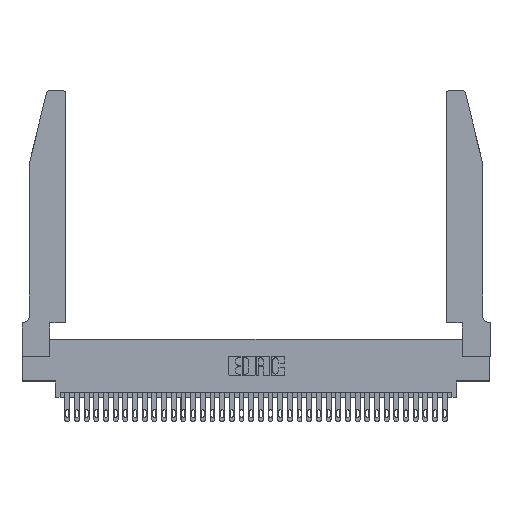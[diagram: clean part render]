
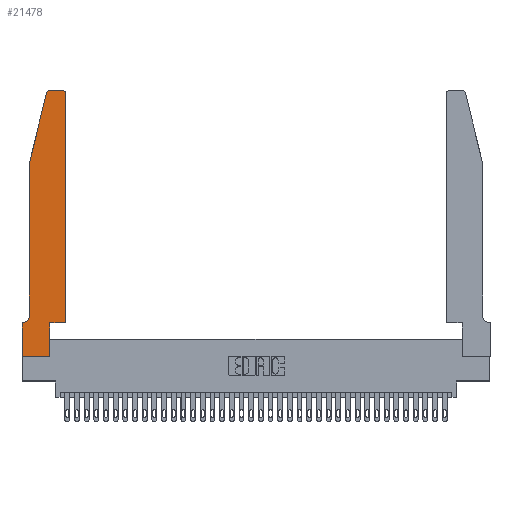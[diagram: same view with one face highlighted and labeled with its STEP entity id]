
A CAD part, top view. The second image highlights one B-rep face of the part: STEP entity #21478.
In plain terms, the highlighted planar face has unit normal (0, 0, 1).
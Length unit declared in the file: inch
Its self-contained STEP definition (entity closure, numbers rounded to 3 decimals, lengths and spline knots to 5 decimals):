
#1144 = CARTESIAN_POINT ( 'NONE',  ( 0.0755, 2., 0.37 ) ) ;
#1197 = DIRECTION ( 'NONE',  ( 0., 0., 1. ) ) ;
#1630 = CARTESIAN_POINT ( 'NONE',  ( 0., 0.35, 0.37 ) ) ;
#1974 = VECTOR ( 'NONE', #9577, 39.37008 ) ;
#2149 = CARTESIAN_POINT ( 'NONE',  ( 0., 0.35, 0.37 ) ) ;
#2601 = VECTOR ( 'NONE', #29135, 39.37008 ) ;
#3172 = LINE ( 'NONE', #26441, #6230 ) ;
#3284 = CARTESIAN_POINT ( 'NONE',  ( 0.4505, 0.35, 0.37 ) ) ;
#3380 = ORIENTED_EDGE ( 'NONE', *, *, #22444, .T. ) ;
#3464 = AXIS2_PLACEMENT_3D ( 'NONE', #7339, #1197, #35227 ) ;
#3904 = CARTESIAN_POINT ( 'NONE',  ( 0.2865, 0.35, 0.37 ) ) ;
#4196 = LINE ( 'NONE', #18011, #1974 ) ;
#5379 = PLANE ( 'NONE',  #22973 ) ;
#5857 = CIRCLE ( 'NONE', #3464, 0.03 ) ;
#5936 = EDGE_CURVE ( 'NONE', #6844, #31489, #5857, .T. ) ;
#6117 = DIRECTION ( 'NONE',  ( 1., 0., 0. ) ) ;
#6230 = VECTOR ( 'NONE', #15509, 39.37008 ) ;
#6342 = LINE ( 'NONE', #3904, #34104 ) ;
#6406 = CARTESIAN_POINT ( 'NONE',  ( 0.0755, 0.35, 0.37 ) ) ;
#6636 = CARTESIAN_POINT ( 'NONE',  ( 0.2865, 0., 0.37 ) ) ;
#6844 = VERTEX_POINT ( 'NONE', #32218 ) ;
#7339 = CARTESIAN_POINT ( 'NONE',  ( 0.284, 2.72, 0.37 ) ) ;
#7535 = VERTEX_POINT ( 'NONE', #23730 ) ;
#8010 = DIRECTION ( 'NONE',  ( 1., 0., 0. ) ) ;
#8126 = VERTEX_POINT ( 'NONE', #1144 ) ;
#8250 = DIRECTION ( 'NONE',  ( 0., 0., 1. ) ) ;
#8351 = VERTEX_POINT ( 'NONE', #29211 ) ;
#9406 = VERTEX_POINT ( 'NONE', #23755 ) ;
#9577 = DIRECTION ( 'NONE',  ( 1., 0., 0. ) ) ;
#9716 = ORIENTED_EDGE ( 'NONE', *, *, #28370, .T. ) ;
#9915 = CARTESIAN_POINT ( 'NONE',  ( 0.4505, 0.35, 0.37 ) ) ;
#10069 = LINE ( 'NONE', #31691, #2601 ) ;
#10891 = CARTESIAN_POINT ( 'NONE',  ( 0., 0., 0.37 ) ) ;
#11590 = FACE_OUTER_BOUND ( 'NONE', #28052, .T. ) ;
#11709 = VERTEX_POINT ( 'NONE', #1630 ) ;
#12345 = VECTOR ( 'NONE', #21558, 39.37008 ) ;
#12691 = DIRECTION ( 'NONE',  ( -0.239, -0.971, 0. ) ) ;
#12763 = LINE ( 'NONE', #6406, #22430 ) ;
#13063 = DIRECTION ( 'NONE',  ( 1., 0., 0. ) ) ;
#13065 = DIRECTION ( 'NONE',  ( 0., -1., 0. ) ) ;
#14072 = EDGE_CURVE ( 'NONE', #11709, #19866, #30857, .T. ) ;
#14424 = CARTESIAN_POINT ( 'NONE',  ( 0.0055, 0.35, 0.37 ) ) ;
#14879 = EDGE_CURVE ( 'NONE', #31489, #8126, #31200, .T. ) ;
#15509 = DIRECTION ( 'NONE',  ( -1., 0., 0. ) ) ;
#15638 = ORIENTED_EDGE ( 'NONE', *, *, #31972, .T. ) ;
#15720 = CARTESIAN_POINT ( 'NONE',  ( 0.4205, 2.72, 0.37 ) ) ;
#16118 = VERTEX_POINT ( 'NONE', #6636 ) ;
#16287 = DIRECTION ( 'NONE',  ( -1., 0., 0. ) ) ;
#16660 = EDGE_CURVE ( 'NONE', #27530, #11709, #12763, .T. ) ;
#16919 = AXIS2_PLACEMENT_3D ( 'NONE', #27986, #36015, #16287 ) ;
#17654 = EDGE_CURVE ( 'NONE', #29062, #9406, #10069, .T. ) ;
#17869 = EDGE_CURVE ( 'NONE', #8126, #7535, #34656, .T. ) ;
#18011 = CARTESIAN_POINT ( 'NONE',  ( 0., 0., 0.37 ) ) ;
#19534 = ORIENTED_EDGE ( 'NONE', *, *, #16660, .T. ) ;
#19610 = VERTEX_POINT ( 'NONE', #35198 ) ;
#19866 = VERTEX_POINT ( 'NONE', #10891 ) ;
#20175 = AXIS2_PLACEMENT_3D ( 'NONE', #15720, #27076, #13063 ) ;
#20528 = VECTOR ( 'NONE', #13065, 39.37008 ) ;
#20540 = LINE ( 'NONE', #3284, #21416 ) ;
#21416 = VECTOR ( 'NONE', #6117, 39.37008 ) ;
#21478 = ADVANCED_FACE ( 'NONE', ( #11590 ), #5379, .T. ) ;
#21558 = DIRECTION ( 'NONE',  ( 0., -1., 0. ) ) ;
#22140 = EDGE_CURVE ( 'NONE', #9406, #8351, #33224, .T. ) ;
#22430 = VECTOR ( 'NONE', #26090, 39.37008 ) ;
#22444 = EDGE_CURVE ( 'NONE', #16118, #19610, #6342, .T. ) ;
#22973 = AXIS2_PLACEMENT_3D ( 'NONE', #2149, #8250, #8010 ) ;
#23157 = ORIENTED_EDGE ( 'NONE', *, *, #5936, .T. ) ;
#23730 = CARTESIAN_POINT ( 'NONE',  ( 0.0755, 0.42, 0.37 ) ) ;
#23755 = CARTESIAN_POINT ( 'NONE',  ( 0.4505, 2.72, 0.37 ) ) ;
#23951 = ORIENTED_EDGE ( 'NONE', *, *, #17869, .T. ) ;
#24337 = CARTESIAN_POINT ( 'NONE',  ( 0.25487, 2.72718, 0.37 ) ) ;
#24645 = ORIENTED_EDGE ( 'NONE', *, *, #22140, .T. ) ;
#24743 = ORIENTED_EDGE ( 'NONE', *, *, #35001, .T. ) ;
#26090 = DIRECTION ( 'NONE',  ( -1., 0., 0. ) ) ;
#26441 = CARTESIAN_POINT ( 'NONE',  ( 0.2605, 2.75, 0.37 ) ) ;
#26535 = DIRECTION ( 'NONE',  ( 0., 1., 0. ) ) ;
#26702 = CARTESIAN_POINT ( 'NONE',  ( 0.0755, 2., 0.37 ) ) ;
#27076 = DIRECTION ( 'NONE',  ( 0., 0., 1. ) ) ;
#27530 = VERTEX_POINT ( 'NONE', #14424 ) ;
#27573 = ORIENTED_EDGE ( 'NONE', *, *, #14072, .T. ) ;
#27986 = CARTESIAN_POINT ( 'NONE',  ( 0.0055, 0.42, 0.37 ) ) ;
#28052 = EDGE_LOOP ( 'NONE', ( #35125, #23157, #31276, #23951, #24743, #19534, #27573, #9716, #3380, #15638, #34528, #24645 ) ) ;
#28370 = EDGE_CURVE ( 'NONE', #19866, #16118, #4196, .T. ) ;
#29062 = VERTEX_POINT ( 'NONE', #9915 ) ;
#29135 = DIRECTION ( 'NONE',  ( 0., 1., 0. ) ) ;
#29211 = CARTESIAN_POINT ( 'NONE',  ( 0.4205, 2.75, 0.37 ) ) ;
#29752 = EDGE_CURVE ( 'NONE', #8351, #6844, #3172, .T. ) ;
#30801 = VECTOR ( 'NONE', #12691, 39.37008 ) ;
#30857 = LINE ( 'NONE', #32641, #12345 ) ;
#31200 = LINE ( 'NONE', #26702, #30801 ) ;
#31276 = ORIENTED_EDGE ( 'NONE', *, *, #14879, .T. ) ;
#31489 = VERTEX_POINT ( 'NONE', #24337 ) ;
#31691 = CARTESIAN_POINT ( 'NONE',  ( 0.4505, 0.35, 0.37 ) ) ;
#31972 = EDGE_CURVE ( 'NONE', #19610, #29062, #20540, .T. ) ;
#32218 = CARTESIAN_POINT ( 'NONE',  ( 0.284, 2.75, 0.37 ) ) ;
#32641 = CARTESIAN_POINT ( 'NONE',  ( 0., 0., 0.37 ) ) ;
#33224 = CIRCLE ( 'NONE', #20175, 0.03 ) ;
#34104 = VECTOR ( 'NONE', #26535, 39.37008 ) ;
#34528 = ORIENTED_EDGE ( 'NONE', *, *, #17654, .T. ) ;
#34656 = LINE ( 'NONE', #35717, #20528 ) ;
#34894 = CIRCLE ( 'NONE', #16919, 0.07 ) ;
#35001 = EDGE_CURVE ( 'NONE', #7535, #27530, #34894, .T. ) ;
#35125 = ORIENTED_EDGE ( 'NONE', *, *, #29752, .T. ) ;
#35198 = CARTESIAN_POINT ( 'NONE',  ( 0.2865, 0.35, 0.37 ) ) ;
#35227 = DIRECTION ( 'NONE',  ( 1., 0., 0. ) ) ;
#35717 = CARTESIAN_POINT ( 'NONE',  ( 0.0755, 2., 0.37 ) ) ;
#36015 = DIRECTION ( 'NONE',  ( 0., 0., -1. ) ) ;
